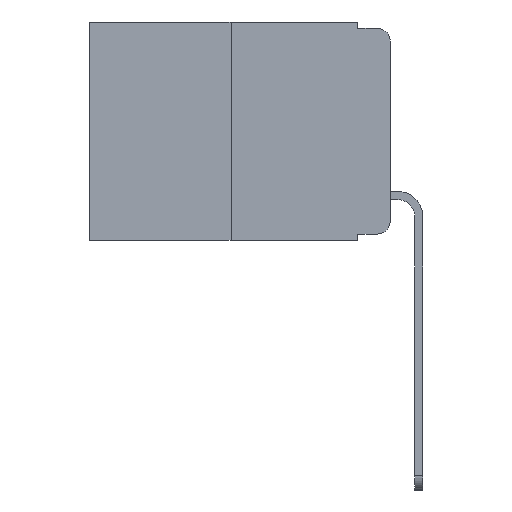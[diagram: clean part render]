
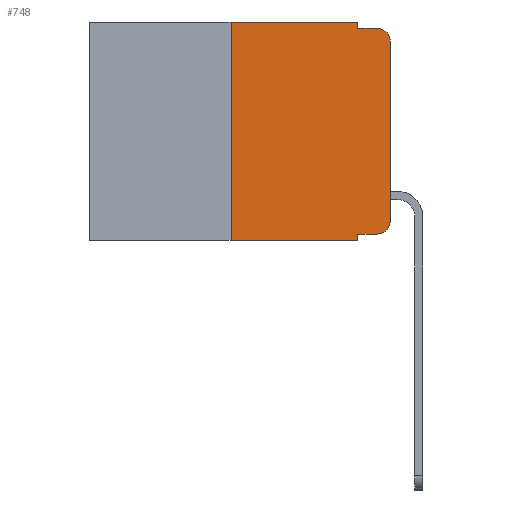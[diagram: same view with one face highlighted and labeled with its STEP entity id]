
A CAD part, left-side view. The second image highlights one B-rep face of the part: STEP entity #748.
In plain terms, the highlighted planar face has unit normal (-1, 0, 0).
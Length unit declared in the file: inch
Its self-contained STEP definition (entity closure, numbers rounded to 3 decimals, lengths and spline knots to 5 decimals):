
#123 = DIRECTION ( 'NONE',  ( 0., -1., 0. ) ) ;
#356 = VECTOR ( 'NONE', #6383, 39.37008 ) ;
#477 = PLANE ( 'NONE',  #14458 ) ;
#535 = LINE ( 'NONE', #3948, #18103 ) ;
#638 = CARTESIAN_POINT ( 'NONE',  ( 0., 0.473, 0. ) ) ;
#748 = ADVANCED_FACE ( 'NONE', ( #23268 ), #477, .F. ) ;
#751 = ORIENTED_EDGE ( 'NONE', *, *, #22521, .F. ) ;
#1301 = LINE ( 'NONE', #16965, #21057 ) ;
#1697 = LINE ( 'NONE', #21630, #23287 ) ;
#1708 = EDGE_CURVE ( 'NONE', #7004, #11215, #1918, .T. ) ;
#1743 = EDGE_CURVE ( 'NONE', #11663, #2497, #6234, .T. ) ;
#1918 = CIRCLE ( 'NONE', #7828, 0.02 ) ;
#1956 = EDGE_CURVE ( 'NONE', #11215, #10160, #23505, .T. ) ;
#2497 = VERTEX_POINT ( 'NONE', #22831 ) ;
#2749 = EDGE_CURVE ( 'NONE', #10160, #22237, #13808, .T. ) ;
#3107 = EDGE_CURVE ( 'NONE', #23306, #10530, #10411, .T. ) ;
#3319 = CARTESIAN_POINT ( 'NONE',  ( 0., 0., 0. ) ) ;
#3535 = VERTEX_POINT ( 'NONE', #16538 ) ;
#3702 = DIRECTION ( 'NONE',  ( 0., 0., -1. ) ) ;
#3793 = VECTOR ( 'NONE', #16901, 39.37008 ) ;
#3948 = CARTESIAN_POINT ( 'NONE',  ( 0., 0.473, 0. ) ) ;
#4014 = ORIENTED_EDGE ( 'NONE', *, *, #23293, .F. ) ;
#4259 = DIRECTION ( 'NONE',  ( -1., 0., 0. ) ) ;
#4273 = EDGE_CURVE ( 'NONE', #3535, #11972, #22389, .T. ) ;
#4413 = DIRECTION ( 'NONE',  ( 0., 0., -1. ) ) ;
#5045 = EDGE_CURVE ( 'NONE', #3535, #7004, #1697, .T. ) ;
#6122 = ORIENTED_EDGE ( 'NONE', *, *, #4273, .F. ) ;
#6234 = LINE ( 'NONE', #14061, #356 ) ;
#6383 = DIRECTION ( 'NONE',  ( 0., 0., 1. ) ) ;
#6509 = DIRECTION ( 'NONE',  ( 0., 0., -1. ) ) ;
#6716 = LINE ( 'NONE', #14298, #22097 ) ;
#6829 = ORIENTED_EDGE ( 'NONE', *, *, #1956, .T. ) ;
#6942 = ORIENTED_EDGE ( 'NONE', *, *, #3107, .F. ) ;
#7004 = VERTEX_POINT ( 'NONE', #18164 ) ;
#7331 = CARTESIAN_POINT ( 'NONE',  ( 0., 0.02, -0.01 ) ) ;
#7475 = DIRECTION ( 'NONE',  ( 0., 0., -1. ) ) ;
#7678 = CARTESIAN_POINT ( 'NONE',  ( 0., 0.051, 0. ) ) ;
#7828 = AXIS2_PLACEMENT_3D ( 'NONE', #10170, #4259, #4413 ) ;
#10160 = VERTEX_POINT ( 'NONE', #23715 ) ;
#10170 = CARTESIAN_POINT ( 'NONE',  ( 0., 0.02, -0.313 ) ) ;
#10411 = LINE ( 'NONE', #7678, #11031 ) ;
#10458 = CARTESIAN_POINT ( 'NONE',  ( 0., 0.051, -0.343 ) ) ;
#10530 = VERTEX_POINT ( 'NONE', #20956 ) ;
#10568 = CARTESIAN_POINT ( 'NONE',  ( 0., 0., -0.313 ) ) ;
#11031 = VECTOR ( 'NONE', #3702, 39.37008 ) ;
#11215 = VERTEX_POINT ( 'NONE', #10568 ) ;
#11247 = DIRECTION ( 'NONE',  ( 0., 0., -1. ) ) ;
#11663 = VERTEX_POINT ( 'NONE', #12209 ) ;
#11972 = VERTEX_POINT ( 'NONE', #10458 ) ;
#12209 = CARTESIAN_POINT ( 'NONE',  ( 0., 0.25, -0.343 ) ) ;
#12477 = DIRECTION ( 'NONE',  ( 1., 0., 0. ) ) ;
#13808 = CIRCLE ( 'NONE', #14153, 0.02 ) ;
#14061 = CARTESIAN_POINT ( 'NONE',  ( 0., 0.25, 0. ) ) ;
#14153 = AXIS2_PLACEMENT_3D ( 'NONE', #19980, #14921, #11247 ) ;
#14298 = CARTESIAN_POINT ( 'NONE',  ( 0., 0.051, -0.01 ) ) ;
#14458 = AXIS2_PLACEMENT_3D ( 'NONE', #638, #12477, #6509 ) ;
#14921 = DIRECTION ( 'NONE',  ( -1., 0., 0. ) ) ;
#15199 = DIRECTION ( 'NONE',  ( 0., -1., 0. ) ) ;
#15284 = ORIENTED_EDGE ( 'NONE', *, *, #2749, .T. ) ;
#15748 = ORIENTED_EDGE ( 'NONE', *, *, #5045, .T. ) ;
#16538 = CARTESIAN_POINT ( 'NONE',  ( 0., 0.051, -0.333 ) ) ;
#16901 = DIRECTION ( 'NONE',  ( 0., 0., 1. ) ) ;
#16965 = CARTESIAN_POINT ( 'NONE',  ( 0., 0.473, -0.343 ) ) ;
#17165 = VECTOR ( 'NONE', #7475, 39.37008 ) ;
#17660 = DIRECTION ( 'NONE',  ( 0., -1., 0. ) ) ;
#17748 = ORIENTED_EDGE ( 'NONE', *, *, #1743, .F. ) ;
#18103 = VECTOR ( 'NONE', #123, 39.37008 ) ;
#18164 = CARTESIAN_POINT ( 'NONE',  ( 0., 0.02, -0.333 ) ) ;
#19972 = EDGE_LOOP ( 'NONE', ( #6829, #15284, #4014, #6942, #751, #17748, #24288, #6122, #15748, #24334 ) ) ;
#19980 = CARTESIAN_POINT ( 'NONE',  ( 0., 0.02, -0.03 ) ) ;
#20246 = CARTESIAN_POINT ( 'NONE',  ( 0., 0.051, 0. ) ) ;
#20375 = EDGE_CURVE ( 'NONE', #11663, #11972, #1301, .T. ) ;
#20517 = DIRECTION ( 'NONE',  ( 0., -1., 0. ) ) ;
#20956 = CARTESIAN_POINT ( 'NONE',  ( 0., 0.051, -0.01 ) ) ;
#21057 = VECTOR ( 'NONE', #15199, 39.37008 ) ;
#21415 = CARTESIAN_POINT ( 'NONE',  ( 0., 0.051, 0. ) ) ;
#21630 = CARTESIAN_POINT ( 'NONE',  ( 0., 0.051, -0.333 ) ) ;
#22097 = VECTOR ( 'NONE', #20517, 39.37008 ) ;
#22237 = VERTEX_POINT ( 'NONE', #7331 ) ;
#22389 = LINE ( 'NONE', #21415, #17165 ) ;
#22521 = EDGE_CURVE ( 'NONE', #2497, #23306, #535, .T. ) ;
#22831 = CARTESIAN_POINT ( 'NONE',  ( 0., 0.25, 0. ) ) ;
#23268 = FACE_OUTER_BOUND ( 'NONE', #19972, .T. ) ;
#23287 = VECTOR ( 'NONE', #17660, 39.37008 ) ;
#23293 = EDGE_CURVE ( 'NONE', #10530, #22237, #6716, .T. ) ;
#23306 = VERTEX_POINT ( 'NONE', #20246 ) ;
#23505 = LINE ( 'NONE', #3319, #3793 ) ;
#23715 = CARTESIAN_POINT ( 'NONE',  ( 0., 0., -0.03 ) ) ;
#24288 = ORIENTED_EDGE ( 'NONE', *, *, #20375, .T. ) ;
#24334 = ORIENTED_EDGE ( 'NONE', *, *, #1708, .T. ) ;
